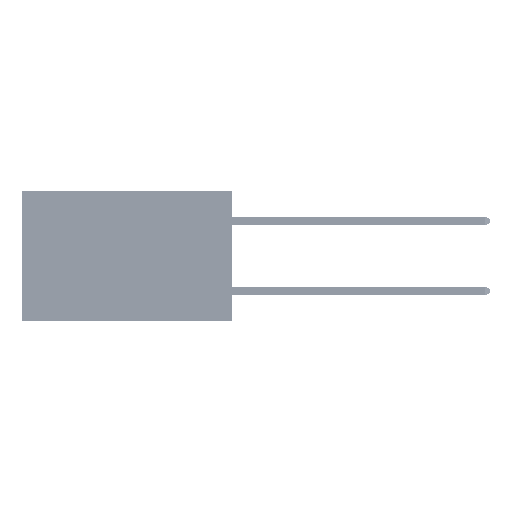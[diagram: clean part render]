
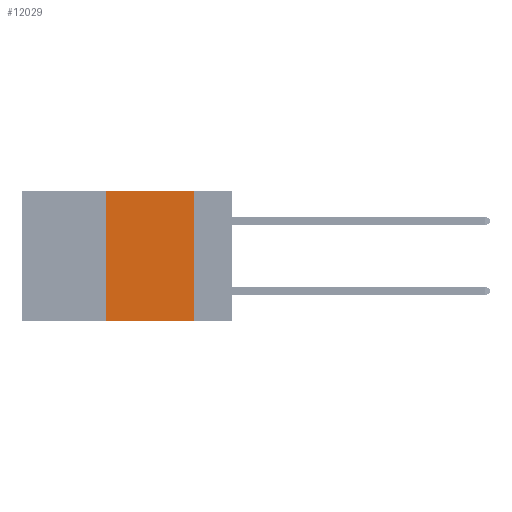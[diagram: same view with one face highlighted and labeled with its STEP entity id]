
A CAD part, left-side view. The second image highlights one B-rep face of the part: STEP entity #12029.
In plain terms, the highlighted planar face has unit normal (-1, 0, 0).
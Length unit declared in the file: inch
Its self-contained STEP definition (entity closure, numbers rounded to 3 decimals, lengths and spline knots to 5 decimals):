
#456 = AXIS2_PLACEMENT_3D ( 'NONE', #31941, #47443, #24932 ) ;
#2448 = FACE_OUTER_BOUND ( 'NONE', #4665, .T. ) ;
#2590 = EDGE_CURVE ( 'NONE', #15096, #29079, #49105, .T. ) ;
#4665 = EDGE_LOOP ( 'NONE', ( #33996, #34313, #7894, #5377 ) ) ;
#5377 = ORIENTED_EDGE ( 'NONE', *, *, #44054, .T. ) ;
#6803 = VECTOR ( 'NONE', #42186, 39.37008 ) ;
#7541 = CARTESIAN_POINT ( 'NONE',  ( 0., 0.6, 0. ) ) ;
#7894 = ORIENTED_EDGE ( 'NONE', *, *, #2590, .F. ) ;
#12029 = ADVANCED_FACE ( 'NONE', ( #2448 ), #22245, .F. ) ;
#12138 = VECTOR ( 'NONE', #39364, 39.37008 ) ;
#12449 = CARTESIAN_POINT ( 'NONE',  ( 0., 0.6, -0.37 ) ) ;
#14365 = CARTESIAN_POINT ( 'NONE',  ( 0., 0.36, -0.37 ) ) ;
#15096 = VERTEX_POINT ( 'NONE', #14365 ) ;
#15618 = VECTOR ( 'NONE', #20586, 39.37008 ) ;
#19677 = VERTEX_POINT ( 'NONE', #44202 ) ;
#20586 = DIRECTION ( 'NONE',  ( 0., -1., 0. ) ) ;
#22003 = CARTESIAN_POINT ( 'NONE',  ( 0., 0.11, 0. ) ) ;
#22245 = PLANE ( 'NONE',  #456 ) ;
#22323 = CARTESIAN_POINT ( 'NONE',  ( 0., 0.11, 0. ) ) ;
#23420 = VERTEX_POINT ( 'NONE', #22003 ) ;
#23450 = VECTOR ( 'NONE', #42961, 39.37008 ) ;
#23894 = CARTESIAN_POINT ( 'NONE',  ( 0., 0.36, 0. ) ) ;
#24932 = DIRECTION ( 'NONE',  ( 0., 0., -1. ) ) ;
#28925 = EDGE_CURVE ( 'NONE', #23420, #19677, #42344, .T. ) ;
#29079 = VERTEX_POINT ( 'NONE', #23894 ) ;
#31941 = CARTESIAN_POINT ( 'NONE',  ( 0., 0.6, 0. ) ) ;
#33996 = ORIENTED_EDGE ( 'NONE', *, *, #28925, .F. ) ;
#34224 = CARTESIAN_POINT ( 'NONE',  ( 0., 0.36, 0. ) ) ;
#34313 = ORIENTED_EDGE ( 'NONE', *, *, #36336, .F. ) ;
#36336 = EDGE_CURVE ( 'NONE', #29079, #23420, #38012, .T. ) ;
#38012 = LINE ( 'NONE', #7541, #12138 ) ;
#39364 = DIRECTION ( 'NONE',  ( 0., -1., 0. ) ) ;
#42186 = DIRECTION ( 'NONE',  ( 0., 0., 1. ) ) ;
#42344 = LINE ( 'NONE', #22323, #23450 ) ;
#42961 = DIRECTION ( 'NONE',  ( 0., 0., -1. ) ) ;
#44054 = EDGE_CURVE ( 'NONE', #15096, #19677, #49133, .T. ) ;
#44202 = CARTESIAN_POINT ( 'NONE',  ( 0., 0.11, -0.37 ) ) ;
#47443 = DIRECTION ( 'NONE',  ( 1., 0., 0. ) ) ;
#49105 = LINE ( 'NONE', #34224, #6803 ) ;
#49133 = LINE ( 'NONE', #12449, #15618 ) ;
